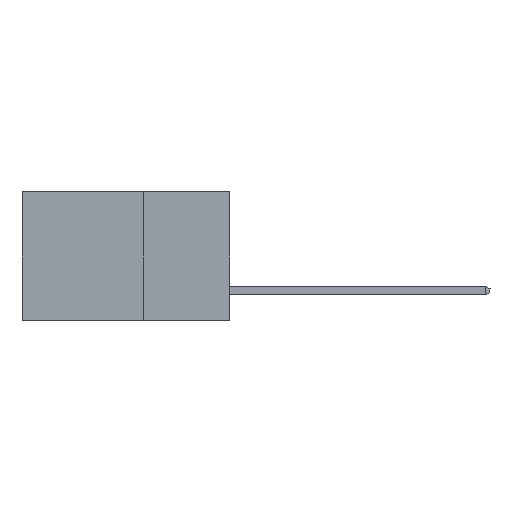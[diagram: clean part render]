
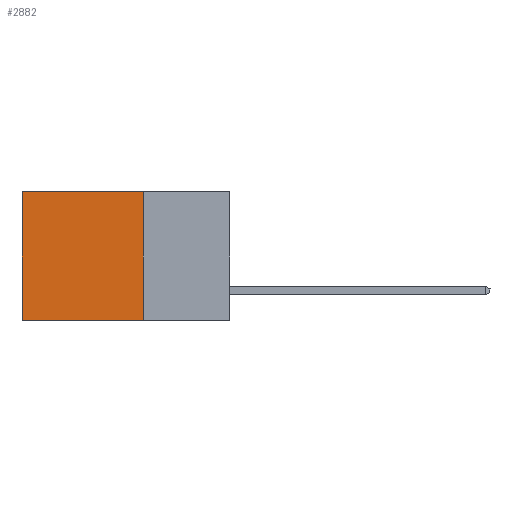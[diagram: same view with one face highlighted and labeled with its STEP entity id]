
A CAD part, left-side view. The second image highlights one B-rep face of the part: STEP entity #2882.
In plain terms, the highlighted planar face has unit normal (-1, 0, 0).
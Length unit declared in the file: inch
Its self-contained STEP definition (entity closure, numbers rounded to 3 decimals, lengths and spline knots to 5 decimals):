
#118 = AXIS2_PLACEMENT_3D ( 'NONE', #1284, #7071, #3760 ) ;
#162 = CARTESIAN_POINT ( 'NONE',  ( 0.2615, 0.25, 0. ) ) ;
#208 = LINE ( 'NONE', #8180, #6180 ) ;
#321 = CARTESIAN_POINT ( 'NONE',  ( 0.2615, 0.25, -0.37 ) ) ;
#382 = VECTOR ( 'NONE', #1973, 39.37008 ) ;
#556 = PLANE ( 'NONE',  #118 ) ;
#580 = CARTESIAN_POINT ( 'NONE',  ( 0.2615, 0.6, -0.37 ) ) ;
#714 = CARTESIAN_POINT ( 'NONE',  ( 0.2615, 0.25, -0.37 ) ) ;
#835 = CARTESIAN_POINT ( 'NONE',  ( 0.2615, 0.6, 0. ) ) ;
#1284 = CARTESIAN_POINT ( 'NONE',  ( 0.2615, 0.25, -0.37 ) ) ;
#1384 = VECTOR ( 'NONE', #7830, 39.37008 ) ;
#1973 = DIRECTION ( 'NONE',  ( 0., 1., 0. ) ) ;
#2309 = VERTEX_POINT ( 'NONE', #5068 ) ;
#2354 = EDGE_LOOP ( 'NONE', ( #9691, #8390, #2677, #8569 ) ) ;
#2483 = VERTEX_POINT ( 'NONE', #714 ) ;
#2628 = DIRECTION ( 'NONE',  ( 0., 1., 0. ) ) ;
#2677 = ORIENTED_EDGE ( 'NONE', *, *, #8347, .F. ) ;
#2882 = ADVANCED_FACE ( 'NONE', ( #2974 ), #556, .F. ) ;
#2974 = FACE_OUTER_BOUND ( 'NONE', #2354, .T. ) ;
#3453 = LINE ( 'NONE', #8665, #1384 ) ;
#3596 = EDGE_CURVE ( 'NONE', #2309, #9516, #4253, .T. ) ;
#3760 = DIRECTION ( 'NONE',  ( 0., 0., -1. ) ) ;
#4253 = LINE ( 'NONE', #162, #5625 ) ;
#5049 = VERTEX_POINT ( 'NONE', #580 ) ;
#5068 = CARTESIAN_POINT ( 'NONE',  ( 0.2615, 0.25, 0. ) ) ;
#5625 = VECTOR ( 'NONE', #2628, 39.37008 ) ;
#5841 = LINE ( 'NONE', #321, #382 ) ;
#6180 = VECTOR ( 'NONE', #9740, 39.37008 ) ;
#6724 = EDGE_CURVE ( 'NONE', #9516, #5049, #3453, .T. ) ;
#7071 = DIRECTION ( 'NONE',  ( 1., 0., 0. ) ) ;
#7830 = DIRECTION ( 'NONE',  ( 0., 0., -1. ) ) ;
#8180 = CARTESIAN_POINT ( 'NONE',  ( 0.2615, 0.25, -0.37 ) ) ;
#8347 = EDGE_CURVE ( 'NONE', #2309, #2483, #208, .T. ) ;
#8390 = ORIENTED_EDGE ( 'NONE', *, *, #9597, .F. ) ;
#8569 = ORIENTED_EDGE ( 'NONE', *, *, #3596, .T. ) ;
#8665 = CARTESIAN_POINT ( 'NONE',  ( 0.2615, 0.6, -0.37 ) ) ;
#9516 = VERTEX_POINT ( 'NONE', #835 ) ;
#9597 = EDGE_CURVE ( 'NONE', #2483, #5049, #5841, .T. ) ;
#9691 = ORIENTED_EDGE ( 'NONE', *, *, #6724, .T. ) ;
#9740 = DIRECTION ( 'NONE',  ( 0., 0., -1. ) ) ;
